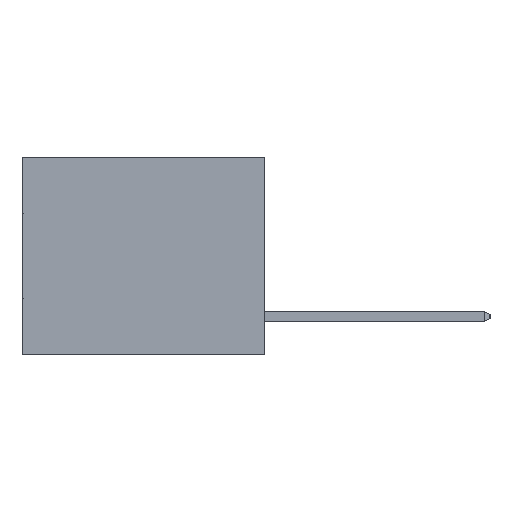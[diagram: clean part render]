
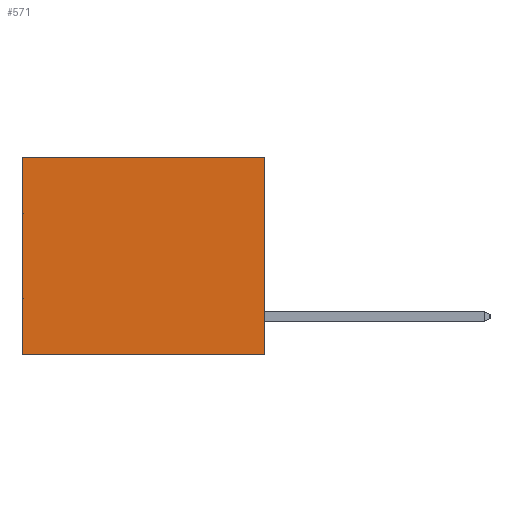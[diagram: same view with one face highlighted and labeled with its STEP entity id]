
A CAD part, left-side view. The second image highlights one B-rep face of the part: STEP entity #571.
In plain terms, the highlighted planar face has unit normal (-1, 0, 0).
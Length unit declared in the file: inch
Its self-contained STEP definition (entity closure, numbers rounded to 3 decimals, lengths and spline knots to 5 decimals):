
#571 = ADVANCED_FACE ( 'NONE', ( #18355 ), #26033, .F. ) ;
#844 = EDGE_CURVE ( 'NONE', #26447, #23420, #1909, .T. ) ;
#863 = DIRECTION ( 'NONE',  ( 0., 1., 0. ) ) ;
#1063 = DIRECTION ( 'NONE',  ( 0., 0., -1. ) ) ;
#1659 = ORIENTED_EDGE ( 'NONE', *, *, #21009, .T. ) ;
#1686 = CARTESIAN_POINT ( 'NONE',  ( 0.3165, 0., -0.49 ) ) ;
#1814 = LINE ( 'NONE', #11240, #10249 ) ;
#1909 = LINE ( 'NONE', #31515, #32722 ) ;
#2744 = CARTESIAN_POINT ( 'NONE',  ( 0.3165, 0., 0. ) ) ;
#2792 = DIRECTION ( 'NONE',  ( 1., 0., 0. ) ) ;
#2856 = LINE ( 'NONE', #28754, #31303 ) ;
#2919 = LINE ( 'NONE', #27148, #7702 ) ;
#3014 = CARTESIAN_POINT ( 'NONE',  ( 0.3165, 0., -0.49 ) ) ;
#6854 = VERTEX_POINT ( 'NONE', #1686 ) ;
#6991 = DIRECTION ( 'NONE',  ( 0., 1., 0. ) ) ;
#7702 = VECTOR ( 'NONE', #6991, 39.37008 ) ;
#8175 = DIRECTION ( 'NONE',  ( 0., 0., -1. ) ) ;
#8578 = CARTESIAN_POINT ( 'NONE',  ( 0.3165, 0.6, 0. ) ) ;
#10249 = VECTOR ( 'NONE', #1063, 39.37008 ) ;
#11240 = CARTESIAN_POINT ( 'NONE',  ( 0.3165, 0., -0.49 ) ) ;
#16760 = ORIENTED_EDGE ( 'NONE', *, *, #18825, .F. ) ;
#18355 = FACE_OUTER_BOUND ( 'NONE', #28011, .T. ) ;
#18825 = EDGE_CURVE ( 'NONE', #26447, #6854, #1814, .T. ) ;
#20649 = ORIENTED_EDGE ( 'NONE', *, *, #20676, .F. ) ;
#20676 = EDGE_CURVE ( 'NONE', #6854, #30040, #2919, .T. ) ;
#20909 = DIRECTION ( 'NONE',  ( 0., 0., -1. ) ) ;
#21009 = EDGE_CURVE ( 'NONE', #23420, #30040, #2856, .T. ) ;
#22489 = AXIS2_PLACEMENT_3D ( 'NONE', #3014, #2792, #20909 ) ;
#23420 = VERTEX_POINT ( 'NONE', #8578 ) ;
#26033 = PLANE ( 'NONE',  #22489 ) ;
#26447 = VERTEX_POINT ( 'NONE', #2744 ) ;
#27148 = CARTESIAN_POINT ( 'NONE',  ( 0.3165, 0., -0.49 ) ) ;
#28011 = EDGE_LOOP ( 'NONE', ( #1659, #20649, #16760, #28256 ) ) ;
#28256 = ORIENTED_EDGE ( 'NONE', *, *, #844, .T. ) ;
#28754 = CARTESIAN_POINT ( 'NONE',  ( 0.3165, 0.6, -0.49 ) ) ;
#30040 = VERTEX_POINT ( 'NONE', #32137 ) ;
#31303 = VECTOR ( 'NONE', #8175, 39.37008 ) ;
#31515 = CARTESIAN_POINT ( 'NONE',  ( 0.3165, 0., 0. ) ) ;
#32137 = CARTESIAN_POINT ( 'NONE',  ( 0.3165, 0.6, -0.49 ) ) ;
#32722 = VECTOR ( 'NONE', #863, 39.37008 ) ;
